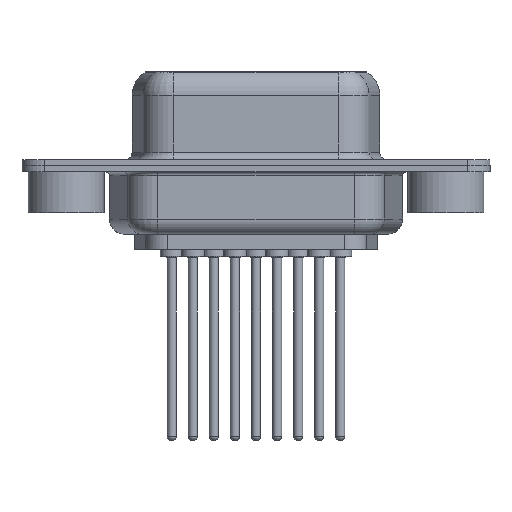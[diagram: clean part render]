
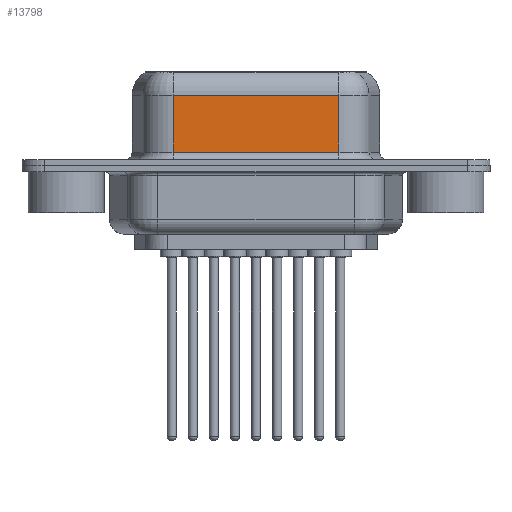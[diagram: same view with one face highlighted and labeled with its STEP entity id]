
A CAD part, front view. The second image highlights one B-rep face of the part: STEP entity #13798.
In plain terms, the highlighted planar face has unit normal (0, -1, 0).
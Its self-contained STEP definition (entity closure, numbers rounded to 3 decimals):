
#502 = CARTESIAN_POINT ( 'NONE',  ( 17.962, -3.95, 4.65 ) ) ;
#1159 = FACE_OUTER_BOUND ( 'NONE', #2712, .T. ) ;
#1922 = DIRECTION ( 'NONE',  ( -1., 0., 0. ) ) ;
#1992 = VECTOR ( 'NONE', #1922, 1000. ) ;
#2160 = CARTESIAN_POINT ( 'NONE',  ( 17.962, -3.95, 4.65 ) ) ;
#2268 = VERTEX_POINT ( 'NONE', #7461 ) ;
#2344 = ORIENTED_EDGE ( 'NONE', *, *, #9196, .T. ) ;
#2712 = EDGE_LOOP ( 'NONE', ( #13588, #2344, #13303, #13238 ) ) ;
#3171 = CARTESIAN_POINT ( 'NONE',  ( 17.962, -3.95, 6.4 ) ) ;
#3665 = DIRECTION ( 'NONE',  ( 0., 1., 0. ) ) ;
#4437 = DIRECTION ( 'NONE',  ( 0., 0., -1. ) ) ;
#4530 = CARTESIAN_POINT ( 'NONE',  ( 7.038, -3.95, 0.9 ) ) ;
#4678 = CARTESIAN_POINT ( 'NONE',  ( 17.962, -3.95, 0.9 ) ) ;
#5940 = DIRECTION ( 'NONE',  ( 0., 0., 1. ) ) ;
#6712 = LINE ( 'NONE', #3171, #8814 ) ;
#7016 = DIRECTION ( 'NONE',  ( 0., 0., -1. ) ) ;
#7353 = PLANE ( 'NONE',  #7359 ) ;
#7359 = AXIS2_PLACEMENT_3D ( 'NONE', #9853, #3665, #5940 ) ;
#7461 = CARTESIAN_POINT ( 'NONE',  ( 7.038, -3.95, 4.65 ) ) ;
#8359 = CARTESIAN_POINT ( 'NONE',  ( 7.038, -3.95, 6.4 ) ) ;
#8587 = VECTOR ( 'NONE', #7016, 1000. ) ;
#8814 = VECTOR ( 'NONE', #4437, 1000. ) ;
#9196 = EDGE_CURVE ( 'NONE', #14671, #2268, #13916, .T. ) ;
#9680 = DIRECTION ( 'NONE',  ( 1., 0., 0. ) ) ;
#9853 = CARTESIAN_POINT ( 'NONE',  ( 17.962, -3.95, 6.4 ) ) ;
#10490 = EDGE_CURVE ( 'NONE', #14671, #14918, #6712, .T. ) ;
#10741 = EDGE_CURVE ( 'NONE', #13586, #14918, #14400, .T. ) ;
#10844 = LINE ( 'NONE', #8359, #8587 ) ;
#11211 = EDGE_CURVE ( 'NONE', #2268, #13586, #10844, .T. ) ;
#13238 = ORIENTED_EDGE ( 'NONE', *, *, #10741, .T. ) ;
#13303 = ORIENTED_EDGE ( 'NONE', *, *, #11211, .T. ) ;
#13586 = VERTEX_POINT ( 'NONE', #4530 ) ;
#13588 = ORIENTED_EDGE ( 'NONE', *, *, #10490, .F. ) ;
#13798 = ADVANCED_FACE ( 'NONE', ( #1159 ), #7353, .F. ) ;
#13916 = LINE ( 'NONE', #2160, #1992 ) ;
#14148 = CARTESIAN_POINT ( 'NONE',  ( 17.962, -3.95, 0.9 ) ) ;
#14313 = VECTOR ( 'NONE', #9680, 1000. ) ;
#14400 = LINE ( 'NONE', #4678, #14313 ) ;
#14671 = VERTEX_POINT ( 'NONE', #502 ) ;
#14918 = VERTEX_POINT ( 'NONE', #14148 ) ;
